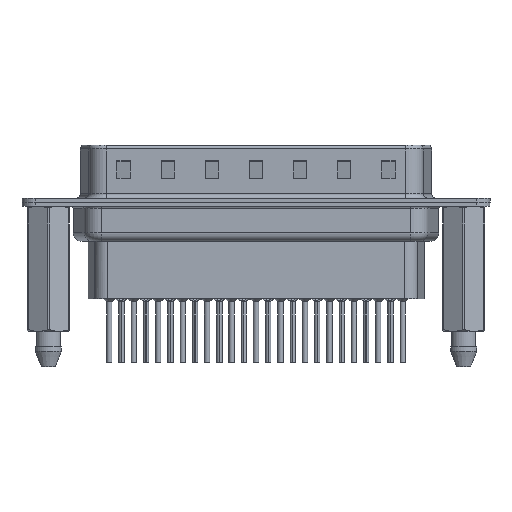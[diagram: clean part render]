
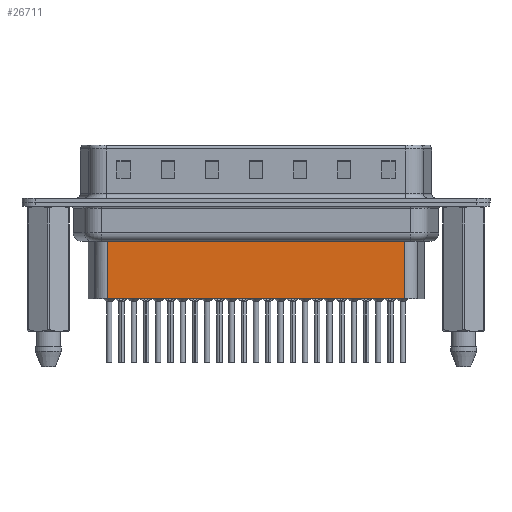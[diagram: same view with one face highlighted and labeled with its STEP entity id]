
A CAD part, front view. The second image highlights one B-rep face of the part: STEP entity #26711.
In plain terms, the highlighted planar face has unit normal (0, -1, 0).
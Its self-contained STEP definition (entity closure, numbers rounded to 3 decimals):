
#43 = DIRECTION ( 'NONE',  ( 1., 0., 0. ) ) ;
#1338 = ORIENTED_EDGE ( 'NONE', *, *, #7645, .T. ) ;
#2047 = EDGE_LOOP ( 'NONE', ( #13932, #14801, #1338, #5641 ) ) ;
#2299 = EDGE_CURVE ( 'NONE', #20894, #12977, #21071, .T. ) ;
#3036 = CARTESIAN_POINT ( 'NONE',  ( 40.344, -3.5, -4.097 ) ) ;
#3564 = DIRECTION ( 'NONE',  ( 0., 0., -1. ) ) ;
#4978 = EDGE_CURVE ( 'NONE', #17040, #20849, #23058, .T. ) ;
#5641 = ORIENTED_EDGE ( 'NONE', *, *, #4978, .F. ) ;
#6385 = CARTESIAN_POINT ( 'NONE',  ( 6.706, -3.5, -3.1 ) ) ;
#6788 = FACE_OUTER_BOUND ( 'NONE', #2047, .T. ) ;
#7645 = EDGE_CURVE ( 'NONE', #12977, #20849, #25706, .T. ) ;
#7984 = CARTESIAN_POINT ( 'NONE',  ( 6.459, -3.5, -4.097 ) ) ;
#8097 = VECTOR ( 'NONE', #25569, 1000. ) ;
#8116 = DIRECTION ( 'NONE',  ( -1., 0., 0. ) ) ;
#11865 = CARTESIAN_POINT ( 'NONE',  ( 40.344, -3.5, -3.1 ) ) ;
#12583 = EDGE_CURVE ( 'NONE', #20894, #17040, #14124, .T. ) ;
#12977 = VERTEX_POINT ( 'NONE', #14093 ) ;
#13932 = ORIENTED_EDGE ( 'NONE', *, *, #12583, .F. ) ;
#14093 = CARTESIAN_POINT ( 'NONE',  ( 6.706, -3.5, -4.097 ) ) ;
#14124 = LINE ( 'NONE', #11865, #23985 ) ;
#14801 = ORIENTED_EDGE ( 'NONE', *, *, #2299, .T. ) ;
#15035 = VECTOR ( 'NONE', #8116, 1000. ) ;
#15382 = PLANE ( 'NONE',  #21089 ) ;
#16587 = CARTESIAN_POINT ( 'NONE',  ( 6.706, -3.5, -10.95 ) ) ;
#16728 = DIRECTION ( 'NONE',  ( -1., 0., 0. ) ) ;
#17040 = VERTEX_POINT ( 'NONE', #19325 ) ;
#17222 = DIRECTION ( 'NONE',  ( 0., -1., 0. ) ) ;
#19325 = CARTESIAN_POINT ( 'NONE',  ( 40.344, -3.5, -10.95 ) ) ;
#20849 = VERTEX_POINT ( 'NONE', #24018 ) ;
#20894 = VERTEX_POINT ( 'NONE', #3036 ) ;
#21071 = LINE ( 'NONE', #7984, #15035 ) ;
#21089 = AXIS2_PLACEMENT_3D ( 'NONE', #6385, #17222, #43 ) ;
#23058 = LINE ( 'NONE', #16587, #25542 ) ;
#23862 = CARTESIAN_POINT ( 'NONE',  ( 6.706, -3.5, -3.1 ) ) ;
#23985 = VECTOR ( 'NONE', #3564, 1000. ) ;
#24018 = CARTESIAN_POINT ( 'NONE',  ( 6.706, -3.5, -10.95 ) ) ;
#25542 = VECTOR ( 'NONE', #16728, 1000. ) ;
#25569 = DIRECTION ( 'NONE',  ( 0., 0., -1. ) ) ;
#25706 = LINE ( 'NONE', #23862, #8097 ) ;
#26711 = ADVANCED_FACE ( 'NONE', ( #6788 ), #15382, .T. ) ;
